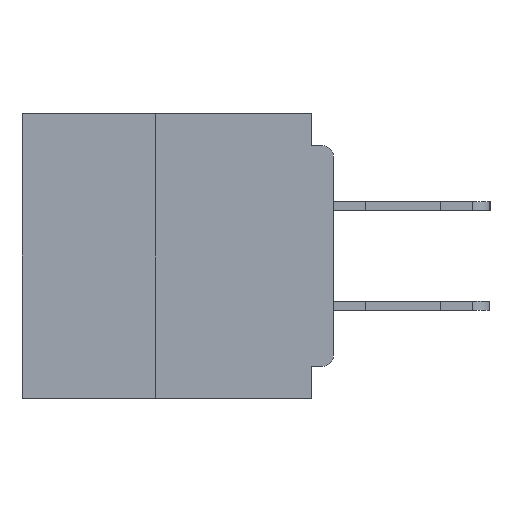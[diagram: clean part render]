
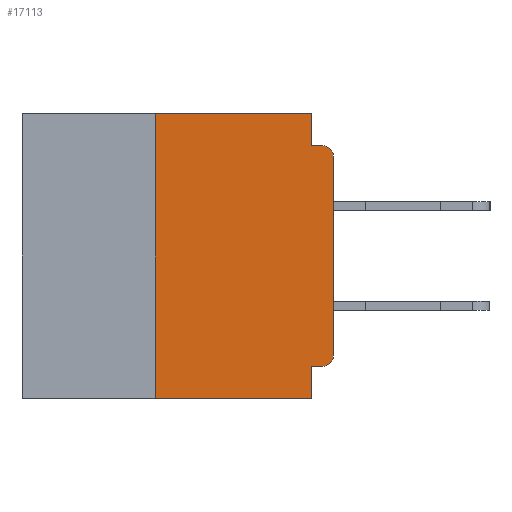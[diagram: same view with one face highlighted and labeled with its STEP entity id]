
A CAD part, left-side view. The second image highlights one B-rep face of the part: STEP entity #17113.
In plain terms, the highlighted planar face has unit normal (-1, 0, 0).
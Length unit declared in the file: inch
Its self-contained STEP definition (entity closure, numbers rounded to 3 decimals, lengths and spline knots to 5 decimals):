
#568 = VECTOR ( 'NONE', #13176, 39.37008 ) ;
#2358 = CARTESIAN_POINT ( 'NONE',  ( 0., 0.031, -0.4 ) ) ;
#2469 = EDGE_CURVE ( 'NONE', #23272, #32386, #52144, .T. ) ;
#3715 = EDGE_CURVE ( 'NONE', #26160, #30409, #11145, .T. ) ;
#5278 = VECTOR ( 'NONE', #52630, 39.37008 ) ;
#6313 = VECTOR ( 'NONE', #19848, 39.37008 ) ;
#6662 = CARTESIAN_POINT ( 'NONE',  ( 0., 0.015, -0.06 ) ) ;
#7396 = CARTESIAN_POINT ( 'NONE',  ( 0., 0.031, -0.4 ) ) ;
#8074 = CIRCLE ( 'NONE', #33372, 0.015 ) ;
#9077 = CARTESIAN_POINT ( 'NONE',  ( 0., 0.031, 0. ) ) ;
#10563 = ORIENTED_EDGE ( 'NONE', *, *, #22195, .F. ) ;
#11145 = CIRCLE ( 'NONE', #37982, 0.015 ) ;
#11327 = DIRECTION ( 'NONE',  ( 0., 0., -1. ) ) ;
#12374 = CARTESIAN_POINT ( 'NONE',  ( 0., 0.437, -0.4 ) ) ;
#12625 = CARTESIAN_POINT ( 'NONE',  ( 0., 0., -0.06 ) ) ;
#12806 = LINE ( 'NONE', #43501, #35741 ) ;
#13176 = DIRECTION ( 'NONE',  ( 0., -1., 0. ) ) ;
#13198 = VERTEX_POINT ( 'NONE', #31122 ) ;
#13643 = PLANE ( 'NONE',  #18804 ) ;
#13656 = DIRECTION ( 'NONE',  ( -1., 0., 0. ) ) ;
#16896 = VECTOR ( 'NONE', #48811, 39.37008 ) ;
#16986 = DIRECTION ( 'NONE',  ( 0., -1., 0. ) ) ;
#17113 = ADVANCED_FACE ( 'NONE', ( #21037 ), #13643, .F. ) ;
#17185 = CARTESIAN_POINT ( 'NONE',  ( 0., 0.015, -0.045 ) ) ;
#18804 = AXIS2_PLACEMENT_3D ( 'NONE', #50360, #22835, #54980 ) ;
#19285 = VERTEX_POINT ( 'NONE', #45439 ) ;
#19517 = LINE ( 'NONE', #24832, #44002 ) ;
#19754 = LINE ( 'NONE', #7396, #16896 ) ;
#19848 = DIRECTION ( 'NONE',  ( 0., 1., 0. ) ) ;
#19941 = ORIENTED_EDGE ( 'NONE', *, *, #37448, .F. ) ;
#20487 = CARTESIAN_POINT ( 'NONE',  ( 0., 0.437, 0. ) ) ;
#21037 = FACE_OUTER_BOUND ( 'NONE', #42341, .T. ) ;
#21399 = LINE ( 'NONE', #12374, #44448 ) ;
#21516 = ORIENTED_EDGE ( 'NONE', *, *, #50670, .F. ) ;
#22195 = EDGE_CURVE ( 'NONE', #13198, #42343, #55196, .T. ) ;
#22835 = DIRECTION ( 'NONE',  ( 1., 0., 0. ) ) ;
#23272 = VERTEX_POINT ( 'NONE', #9077 ) ;
#24832 = CARTESIAN_POINT ( 'NONE',  ( 0., 0.25, -0.4 ) ) ;
#26160 = VERTEX_POINT ( 'NONE', #12625 ) ;
#27185 = EDGE_CURVE ( 'NONE', #19285, #26160, #12806, .T. ) ;
#27652 = VECTOR ( 'NONE', #53442, 39.37008 ) ;
#30228 = ORIENTED_EDGE ( 'NONE', *, *, #59010, .F. ) ;
#30409 = VERTEX_POINT ( 'NONE', #17185 ) ;
#31122 = CARTESIAN_POINT ( 'NONE',  ( 0., 0.015, -0.355 ) ) ;
#32367 = CARTESIAN_POINT ( 'NONE',  ( 0., 0.25, 0. ) ) ;
#32386 = VERTEX_POINT ( 'NONE', #54075 ) ;
#33372 = AXIS2_PLACEMENT_3D ( 'NONE', #41188, #13656, #45798 ) ;
#33844 = ORIENTED_EDGE ( 'NONE', *, *, #2469, .F. ) ;
#35741 = VECTOR ( 'NONE', #48107, 39.37008 ) ;
#36384 = ORIENTED_EDGE ( 'NONE', *, *, #40623, .T. ) ;
#37448 = EDGE_CURVE ( 'NONE', #42343, #51349, #19754, .T. ) ;
#37982 = AXIS2_PLACEMENT_3D ( 'NONE', #6662, #38841, #11327 ) ;
#38770 = ORIENTED_EDGE ( 'NONE', *, *, #44934, .T. ) ;
#38841 = DIRECTION ( 'NONE',  ( -1., 0., 0. ) ) ;
#39012 = ORIENTED_EDGE ( 'NONE', *, *, #40735, .F. ) ;
#40623 = EDGE_CURVE ( 'NONE', #59267, #51349, #21399, .T. ) ;
#40735 = EDGE_CURVE ( 'NONE', #32386, #30409, #50832, .T. ) ;
#41188 = CARTESIAN_POINT ( 'NONE',  ( 0., 0.015, -0.34 ) ) ;
#41994 = LINE ( 'NONE', #20487, #5278 ) ;
#42341 = EDGE_LOOP ( 'NONE', ( #59311, #51981, #39012, #33844, #21516, #30228, #36384, #19941, #10563, #38770 ) ) ;
#42343 = VERTEX_POINT ( 'NONE', #43184 ) ;
#43184 = CARTESIAN_POINT ( 'NONE',  ( 0., 0.031, -0.355 ) ) ;
#43501 = CARTESIAN_POINT ( 'NONE',  ( 0., 0., 0. ) ) ;
#44002 = VECTOR ( 'NONE', #56943, 39.37008 ) ;
#44448 = VECTOR ( 'NONE', #16986, 39.37008 ) ;
#44934 = EDGE_CURVE ( 'NONE', #13198, #19285, #8074, .T. ) ;
#45313 = CARTESIAN_POINT ( 'NONE',  ( 0., 0., -0.045 ) ) ;
#45439 = CARTESIAN_POINT ( 'NONE',  ( 0., 0., -0.34 ) ) ;
#45798 = DIRECTION ( 'NONE',  ( 0., 0., -1. ) ) ;
#48107 = DIRECTION ( 'NONE',  ( 0., 0., 1. ) ) ;
#48811 = DIRECTION ( 'NONE',  ( 0., 0., -1. ) ) ;
#50360 = CARTESIAN_POINT ( 'NONE',  ( 0., 0.437, 0. ) ) ;
#50670 = EDGE_CURVE ( 'NONE', #53776, #23272, #41994, .T. ) ;
#50832 = LINE ( 'NONE', #45313, #568 ) ;
#51349 = VERTEX_POINT ( 'NONE', #2358 ) ;
#51981 = ORIENTED_EDGE ( 'NONE', *, *, #3715, .T. ) ;
#52144 = LINE ( 'NONE', #53578, #27652 ) ;
#52630 = DIRECTION ( 'NONE',  ( 0., -1., 0. ) ) ;
#53442 = DIRECTION ( 'NONE',  ( 0., 0., -1. ) ) ;
#53578 = CARTESIAN_POINT ( 'NONE',  ( 0., 0.031, 0. ) ) ;
#53776 = VERTEX_POINT ( 'NONE', #32367 ) ;
#54075 = CARTESIAN_POINT ( 'NONE',  ( 0., 0.031, -0.045 ) ) ;
#54980 = DIRECTION ( 'NONE',  ( 0., 0., -1. ) ) ;
#55196 = LINE ( 'NONE', #56598, #6313 ) ;
#56598 = CARTESIAN_POINT ( 'NONE',  ( 0., 0., -0.355 ) ) ;
#56943 = DIRECTION ( 'NONE',  ( 0., 0., 1. ) ) ;
#58718 = CARTESIAN_POINT ( 'NONE',  ( 0., 0.25, -0.4 ) ) ;
#59010 = EDGE_CURVE ( 'NONE', #59267, #53776, #19517, .T. ) ;
#59267 = VERTEX_POINT ( 'NONE', #58718 ) ;
#59311 = ORIENTED_EDGE ( 'NONE', *, *, #27185, .T. ) ;
